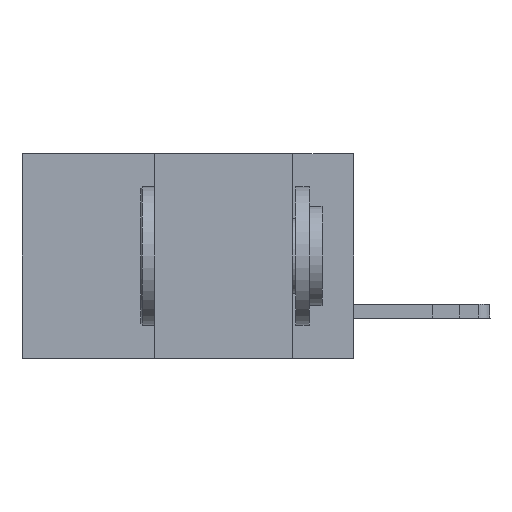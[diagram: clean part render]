
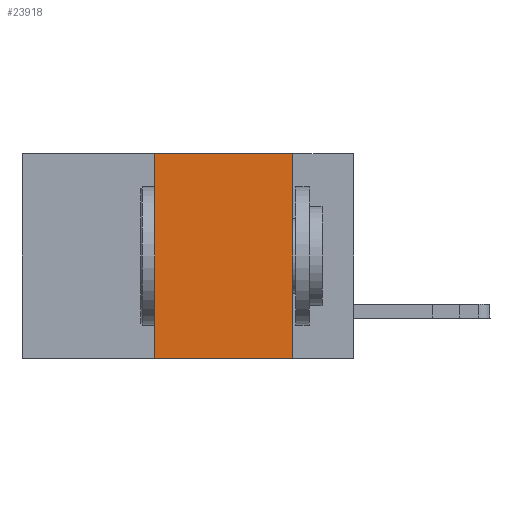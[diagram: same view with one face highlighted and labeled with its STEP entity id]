
A CAD part, left-side view. The second image highlights one B-rep face of the part: STEP entity #23918.
In plain terms, the highlighted planar face has unit normal (-1, 0, 0).
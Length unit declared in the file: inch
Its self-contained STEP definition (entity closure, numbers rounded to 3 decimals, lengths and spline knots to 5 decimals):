
#546 = EDGE_CURVE ( 'NONE', #19048, #8297, #20683, .T. ) ;
#804 = LINE ( 'NONE', #17402, #21517 ) ;
#1041 = CARTESIAN_POINT ( 'NONE',  ( 0., 0.6, 0. ) ) ;
#1303 = ORIENTED_EDGE ( 'NONE', *, *, #546, .F. ) ;
#1803 = EDGE_CURVE ( 'NONE', #3565, #2747, #16362, .T. ) ;
#2747 = VERTEX_POINT ( 'NONE', #11859 ) ;
#2995 = DIRECTION ( 'NONE',  ( 0., -1., 0. ) ) ;
#3393 = LINE ( 'NONE', #14761, #19164 ) ;
#3565 = VERTEX_POINT ( 'NONE', #6250 ) ;
#3652 = EDGE_CURVE ( 'NONE', #8297, #3565, #3393, .T. ) ;
#4555 = DIRECTION ( 'NONE',  ( 0., -1., 0. ) ) ;
#4591 = ORIENTED_EDGE ( 'NONE', *, *, #1803, .F. ) ;
#5868 = ORIENTED_EDGE ( 'NONE', *, *, #16307, .T. ) ;
#6250 = CARTESIAN_POINT ( 'NONE',  ( 0., 0.11, 0. ) ) ;
#7815 = ORIENTED_EDGE ( 'NONE', *, *, #3652, .F. ) ;
#8297 = VERTEX_POINT ( 'NONE', #13092 ) ;
#11432 = DIRECTION ( 'NONE',  ( 0., 0., -1. ) ) ;
#11531 = VECTOR ( 'NONE', #13893, 39.37008 ) ;
#11859 = CARTESIAN_POINT ( 'NONE',  ( 0., 0.11, -0.37 ) ) ;
#13092 = CARTESIAN_POINT ( 'NONE',  ( 0., 0.36, 0. ) ) ;
#13600 = EDGE_LOOP ( 'NONE', ( #4591, #7815, #1303, #5868 ) ) ;
#13800 = CARTESIAN_POINT ( 'NONE',  ( 0., 0.11, 0. ) ) ;
#13893 = DIRECTION ( 'NONE',  ( 0., 0., -1. ) ) ;
#14761 = CARTESIAN_POINT ( 'NONE',  ( 0., 0.6, 0. ) ) ;
#15003 = AXIS2_PLACEMENT_3D ( 'NONE', #1041, #23817, #11432 ) ;
#15421 = DIRECTION ( 'NONE',  ( 0., 0., 1. ) ) ;
#15528 = CARTESIAN_POINT ( 'NONE',  ( 0., 0.36, 0. ) ) ;
#16307 = EDGE_CURVE ( 'NONE', #19048, #2747, #804, .T. ) ;
#16362 = LINE ( 'NONE', #13800, #11531 ) ;
#17402 = CARTESIAN_POINT ( 'NONE',  ( 0., 0.6, -0.37 ) ) ;
#17551 = PLANE ( 'NONE',  #15003 ) ;
#19048 = VERTEX_POINT ( 'NONE', #25147 ) ;
#19164 = VECTOR ( 'NONE', #4555, 39.37008 ) ;
#20683 = LINE ( 'NONE', #15528, #26133 ) ;
#21517 = VECTOR ( 'NONE', #2995, 39.37008 ) ;
#23817 = DIRECTION ( 'NONE',  ( 1., 0., 0. ) ) ;
#23918 = ADVANCED_FACE ( 'NONE', ( #26079 ), #17551, .F. ) ;
#25147 = CARTESIAN_POINT ( 'NONE',  ( 0., 0.36, -0.37 ) ) ;
#26079 = FACE_OUTER_BOUND ( 'NONE', #13600, .T. ) ;
#26133 = VECTOR ( 'NONE', #15421, 39.37008 ) ;
